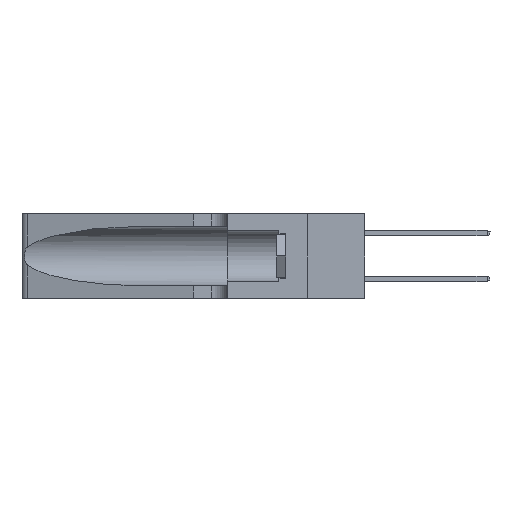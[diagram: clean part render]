
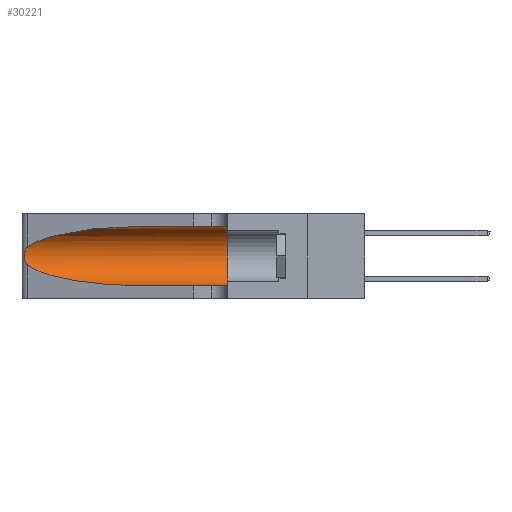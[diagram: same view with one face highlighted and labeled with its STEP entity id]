
A CAD part, left-side view. The second image highlights one B-rep face of the part: STEP entity #30221.
In plain terms, the highlighted cylindrical face has radius 3.308 mm (diameter 6.617 mm), a partial arc.
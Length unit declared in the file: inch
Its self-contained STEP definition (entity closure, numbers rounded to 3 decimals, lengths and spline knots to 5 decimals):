
#368 = CARTESIAN_POINT ( 'NONE',  ( 0.1305, 0.72297, 0.05475 ) ) ;
#1273 = CARTESIAN_POINT ( 'NONE',  ( 0.1305, 1.61858, 0.05475 ) ) ;
#1911 = CARTESIAN_POINT ( 'NONE',  ( 0.1305, 0.72297, 0.05475 ) ) ;
#2649 = DIRECTION ( 'NONE',  ( 0., 0., -1. ) ) ;
#3816 = ORIENTED_EDGE ( 'NONE', *, *, #41121, .T. ) ;
#3849 =( BOUNDED_CURVE ( )  B_SPLINE_CURVE ( 3, ( #41064, #21482, #11936, #1911 ),
 .UNSPECIFIED., .F., .T. ) 
 B_SPLINE_CURVE_WITH_KNOTS ( ( 4, 4 ),
 ( 3.44316, 4.71239 ),
 .UNSPECIFIED. ) 
 CURVE ( )  GEOMETRIC_REPRESENTATION_ITEM ( )  RATIONAL_B_SPLINE_CURVE ( ( 1., 0.87, 0.87, 1. ) ) 
 REPRESENTATION_ITEM ( '' )  );
#3874 = CARTESIAN_POINT ( 'NONE',  ( 0.25639, 1.23186, 0.15144 ) ) ;
#4958 = ORIENTED_EDGE ( 'NONE', *, *, #27988, .F. ) ;
#5276 = CARTESIAN_POINT ( 'NONE',  ( 0.25487, 1.22718, 0.22369 ) ) ;
#5859 = CARTESIAN_POINT ( 'NONE',  ( 0.25487, 1.22718, 0.14631 ) ) ;
#6420 = ORIENTED_EDGE ( 'NONE', *, *, #19828, .T. ) ;
#6530 = FACE_OUTER_BOUND ( 'NONE', #26023, .T. ) ;
#6708 = CARTESIAN_POINT ( 'NONE',  ( 0.25487, 1.22718, 0.22369 ) ) ;
#6947 = CARTESIAN_POINT ( 'NONE',  ( 0.1305, 0.35, 0.185 ) ) ;
#9966 = CARTESIAN_POINT ( 'NONE',  ( 0.26017, 1.23833, 0.17102 ) ) ;
#10307 = CARTESIAN_POINT ( 'NONE',  ( 0.25555, 1.22994, 0.2215 ) ) ;
#10977 = ORIENTED_EDGE ( 'NONE', *, *, #12430, .T. ) ;
#11684 = CARTESIAN_POINT ( 'NONE',  ( 0.2373, 1.15595, 0.28018 ) ) ;
#11936 = CARTESIAN_POINT ( 'NONE',  ( 0.18966, 0.96281, 0.05475 ) ) ;
#12205 = CARTESIAN_POINT ( 'NONE',  ( 0.1305, 0.72297, 0.31525 ) ) ;
#12430 = EDGE_CURVE ( 'NONE', #37155, #29618, #31848, .T. ) ;
#13034 = CARTESIAN_POINT ( 'NONE',  ( 0.25787, 1.23484, 0.2124 ) ) ;
#13389 = CARTESIAN_POINT ( 'NONE',  ( 0.1305, 0.35, 0.05475 ) ) ;
#13787 = AXIS2_PLACEMENT_3D ( 'NONE', #6947, #23574, #23300 ) ;
#14186 = VERTEX_POINT ( 'NONE', #13389 ) ;
#15275 = EDGE_CURVE ( 'NONE', #20598, #25506, #30554, .T. ) ;
#17689 = VECTOR ( 'NONE', #30831, 39.37008 ) ;
#19828 = EDGE_CURVE ( 'NONE', #20598, #37155, #26100, .T. ) ;
#19968 = CARTESIAN_POINT ( 'NONE',  ( 0.26075, 1.23896, 0.19203 ) ) ;
#20598 = VERTEX_POINT ( 'NONE', #12205 ) ;
#21482 = CARTESIAN_POINT ( 'NONE',  ( 0.2373, 1.15595, 0.08982 ) ) ;
#21963 = VECTOR ( 'NONE', #33186, 39.37008 ) ;
#23167 = CARTESIAN_POINT ( 'NONE',  ( 0.1305, 1.61858, 0.31525 ) ) ;
#23300 = DIRECTION ( 'NONE',  ( 0., 0., 1. ) ) ;
#23574 = DIRECTION ( 'NONE',  ( 0., 1., 0. ) ) ;
#24298 = LINE ( 'NONE', #1273, #17689 ) ;
#25069 = CARTESIAN_POINT ( 'NONE',  ( 0.1305, 0.72297, 0.31525 ) ) ;
#25506 = VERTEX_POINT ( 'NONE', #29901 ) ;
#25931 = CARTESIAN_POINT ( 'NONE',  ( 0.25487, 1.22718, 0.14631 ) ) ;
#26023 = EDGE_LOOP ( 'NONE', ( #6420, #10977, #3816, #36924, #4958, #28130 ) ) ;
#26100 =( BOUNDED_CURVE ( )  B_SPLINE_CURVE ( 3, ( #25069, #38103, #11684, #5276 ),
 .UNSPECIFIED., .F., .F. ) 
 B_SPLINE_CURVE_WITH_KNOTS ( ( 4, 4 ),
 ( 1.5708, 2.84003 ),
 .UNSPECIFIED. ) 
 CURVE ( )  GEOMETRIC_REPRESENTATION_ITEM ( )  RATIONAL_B_SPLINE_CURVE ( ( 1., 0.87, 0.87, 1. ) ) 
 REPRESENTATION_ITEM ( '' )  );
#26931 = CARTESIAN_POINT ( 'NONE',  ( 0.25856, 1.23593, 0.16098 ) ) ;
#27988 = EDGE_CURVE ( 'NONE', #25506, #14186, #39569, .T. ) ;
#28130 = ORIENTED_EDGE ( 'NONE', *, *, #15275, .F. ) ;
#29445 = CARTESIAN_POINT ( 'NONE',  ( 0.26075, 1.23896, 0.178 ) ) ;
#29618 = VERTEX_POINT ( 'NONE', #5859 ) ;
#29736 = CARTESIAN_POINT ( 'NONE',  ( 0.25555, 1.22993, 0.14849 ) ) ;
#29901 = CARTESIAN_POINT ( 'NONE',  ( 0.1305, 0.35, 0.31525 ) ) ;
#30221 = ADVANCED_FACE ( 'NONE', ( #6530 ), #31510, .F. ) ;
#30554 = LINE ( 'NONE', #23167, #21963 ) ;
#30772 = EDGE_CURVE ( 'NONE', #35925, #14186, #24298, .T. ) ;
#30831 = DIRECTION ( 'NONE',  ( 0., -1., 0. ) ) ;
#31390 = CARTESIAN_POINT ( 'NONE',  ( 0.25639, 1.23184, 0.21858 ) ) ;
#31510 = CYLINDRICAL_SURFACE ( 'NONE', #32385, 0.13025 ) ;
#31848 = B_SPLINE_CURVE_WITH_KNOTS ( 'NONE', 3,
 ( #41754, #10307, #31390, #13034, #32795, #36240, #19968, #29445, #9966, #26931, #32929, #3874, #29736, #25931 ),
 .UNSPECIFIED., .F., .F.,
 ( 4, 2, 2, 2, 2, 2, 4 ),
 ( 0., 0.00027, 0.00053, 0.00107, 0.0016, 0.00187, 0.00214 ),
 .UNSPECIFIED. ) ;
#32015 = CARTESIAN_POINT ( 'NONE',  ( 0.1305, 1.61858, 0.185 ) ) ;
#32296 = DIRECTION ( 'NONE',  ( 0., -1., 0. ) ) ;
#32385 = AXIS2_PLACEMENT_3D ( 'NONE', #32015, #32296, #2649 ) ;
#32795 = CARTESIAN_POINT ( 'NONE',  ( 0.25854, 1.2359, 0.20912 ) ) ;
#32929 = CARTESIAN_POINT ( 'NONE',  ( 0.25789, 1.23486, 0.15765 ) ) ;
#33186 = DIRECTION ( 'NONE',  ( 0., -1., 0. ) ) ;
#35925 = VERTEX_POINT ( 'NONE', #368 ) ;
#36240 = CARTESIAN_POINT ( 'NONE',  ( 0.26018, 1.23835, 0.19895 ) ) ;
#36924 = ORIENTED_EDGE ( 'NONE', *, *, #30772, .T. ) ;
#37155 = VERTEX_POINT ( 'NONE', #6708 ) ;
#38103 = CARTESIAN_POINT ( 'NONE',  ( 0.18966, 0.96281, 0.31525 ) ) ;
#39569 = CIRCLE ( 'NONE', #13787, 0.13025 ) ;
#41064 = CARTESIAN_POINT ( 'NONE',  ( 0.25487, 1.22718, 0.14631 ) ) ;
#41121 = EDGE_CURVE ( 'NONE', #29618, #35925, #3849, .T. ) ;
#41754 = CARTESIAN_POINT ( 'NONE',  ( 0.25487, 1.22718, 0.22369 ) ) ;
